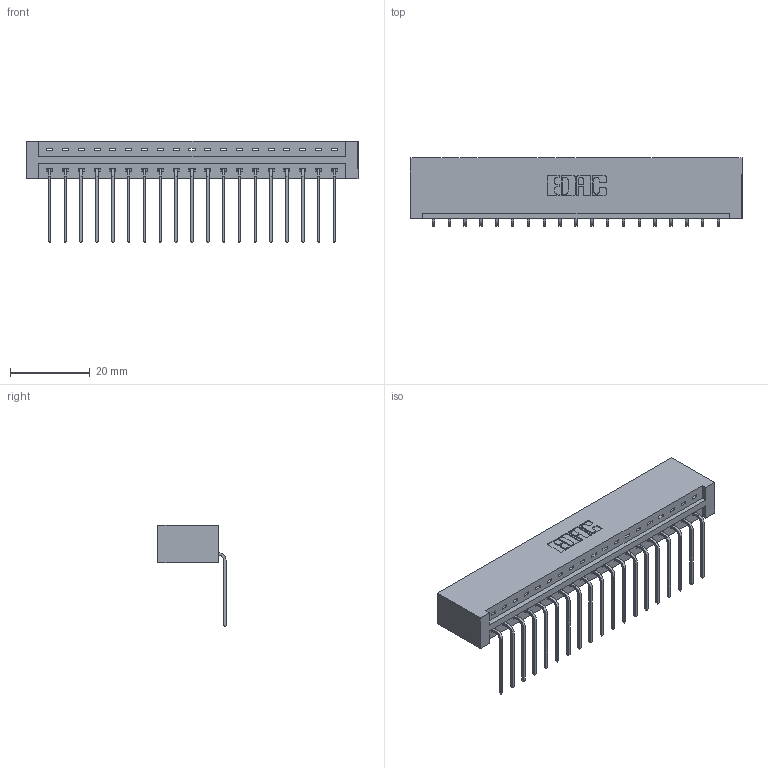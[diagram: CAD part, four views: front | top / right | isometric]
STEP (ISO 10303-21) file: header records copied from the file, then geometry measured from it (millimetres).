
FILE_DESCRIPTION (( 'STEP AP203' ), '1' );
FILE_NAME ('387-019-559-101.STEP', '2019-10-02T21:52:54', ( '' ), ( '' ), 'SwSTEP 2.0', 'SolidWorks 2016', '' );
FILE_SCHEMA (( 'CONFIG_CONTROL_DESIGN' ));
Length unit declared in the file: inch
Products named in the file (3): 337 Part_No Mounting Lugs; 345-292-001_558 559 Tail - 1; 387-019-559-101
Assembly tree (20 placements, depth 2):
  387-019-559-101
    337 Part_No Mounting Lugs
    345-292-001_558 559 Tail - 1  x19
Bounding box: 83.16 x 17.09 x 25.53 mm (x, y, z)
Volume: 9157.2 mm3; surface area: 9705.3 mm2
Topology: 20 solids, 20 shells, 1322 faces, 3973 edges, 2622 vertices
Faces by surface type: plane 978, cylinder 344
Entity records: 16905 total; most frequent: CARTESIAN_POINT 2951, ORIENTED_EDGE 2906, DIRECTION 2523, EDGE_CURVE 1453, LINE 1333, VECTOR 1333, VERTEX_POINT 966, AXIS2_PLACEMENT_3D 595
